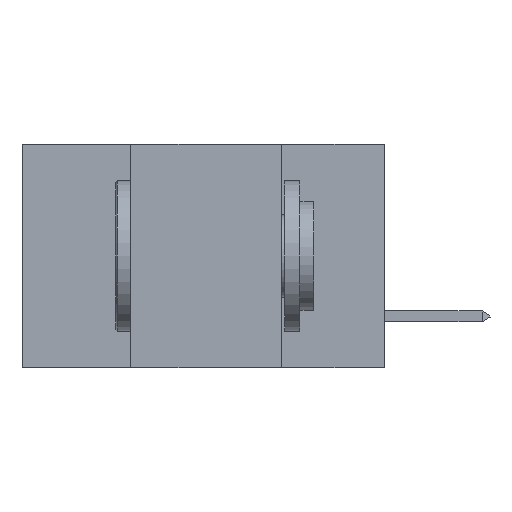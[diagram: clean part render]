
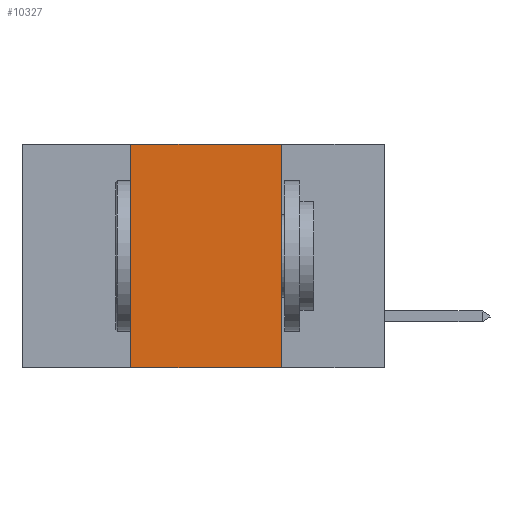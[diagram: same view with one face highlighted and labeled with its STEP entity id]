
A CAD part, left-side view. The second image highlights one B-rep face of the part: STEP entity #10327.
In plain terms, the highlighted planar face has unit normal (-1, 0, 0).
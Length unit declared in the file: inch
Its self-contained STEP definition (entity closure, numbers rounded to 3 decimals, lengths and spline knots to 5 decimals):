
#1090 = LINE ( 'NONE', #38853, #10498 ) ;
#1316 = CARTESIAN_POINT ( 'NONE',  ( 0., 0.17, 0. ) ) ;
#1447 = VECTOR ( 'NONE', #18313, 39.37008 ) ;
#3560 = EDGE_CURVE ( 'NONE', #20925, #28574, #10819, .T. ) ;
#3973 = LINE ( 'NONE', #36783, #27918 ) ;
#5495 = PLANE ( 'NONE',  #9077 ) ;
#6069 = VERTEX_POINT ( 'NONE', #37231 ) ;
#9077 = AXIS2_PLACEMENT_3D ( 'NONE', #22294, #35501, #28710 ) ;
#9488 = DIRECTION ( 'NONE',  ( 0., 0., 1. ) ) ;
#10327 = ADVANCED_FACE ( 'NONE', ( #37668 ), #5495, .F. ) ;
#10498 = VECTOR ( 'NONE', #18824, 39.37008 ) ;
#10819 = LINE ( 'NONE', #1316, #1447 ) ;
#12069 = EDGE_CURVE ( 'NONE', #6069, #20925, #1090, .T. ) ;
#12908 = ORIENTED_EDGE ( 'NONE', *, *, #3560, .F. ) ;
#14451 = EDGE_LOOP ( 'NONE', ( #12908, #34317, #23472, #37001 ) ) ;
#18313 = DIRECTION ( 'NONE',  ( 0., 0., -1. ) ) ;
#18824 = DIRECTION ( 'NONE',  ( 0., -1., 0. ) ) ;
#19358 = CARTESIAN_POINT ( 'NONE',  ( 0., 0.42, -0.37 ) ) ;
#20925 = VERTEX_POINT ( 'NONE', #34745 ) ;
#22017 = EDGE_CURVE ( 'NONE', #40545, #28574, #3973, .T. ) ;
#22294 = CARTESIAN_POINT ( 'NONE',  ( 0., 0.6, 0. ) ) ;
#23304 = CARTESIAN_POINT ( 'NONE',  ( 0., 0.17, -0.37 ) ) ;
#23472 = ORIENTED_EDGE ( 'NONE', *, *, #36933, .F. ) ;
#23726 = DIRECTION ( 'NONE',  ( 0., -1., 0. ) ) ;
#24253 = LINE ( 'NONE', #42965, #26322 ) ;
#26322 = VECTOR ( 'NONE', #9488, 39.37008 ) ;
#27918 = VECTOR ( 'NONE', #23726, 39.37008 ) ;
#28574 = VERTEX_POINT ( 'NONE', #23304 ) ;
#28710 = DIRECTION ( 'NONE',  ( 0., 0., -1. ) ) ;
#34317 = ORIENTED_EDGE ( 'NONE', *, *, #12069, .F. ) ;
#34745 = CARTESIAN_POINT ( 'NONE',  ( 0., 0.17, 0. ) ) ;
#35501 = DIRECTION ( 'NONE',  ( 1., 0., 0. ) ) ;
#36783 = CARTESIAN_POINT ( 'NONE',  ( 0., 0.6, -0.37 ) ) ;
#36933 = EDGE_CURVE ( 'NONE', #40545, #6069, #24253, .T. ) ;
#37001 = ORIENTED_EDGE ( 'NONE', *, *, #22017, .T. ) ;
#37231 = CARTESIAN_POINT ( 'NONE',  ( 0., 0.42, 0. ) ) ;
#37668 = FACE_OUTER_BOUND ( 'NONE', #14451, .T. ) ;
#38853 = CARTESIAN_POINT ( 'NONE',  ( 0., 0.6, 0. ) ) ;
#40545 = VERTEX_POINT ( 'NONE', #19358 ) ;
#42965 = CARTESIAN_POINT ( 'NONE',  ( 0., 0.42, 0. ) ) ;
